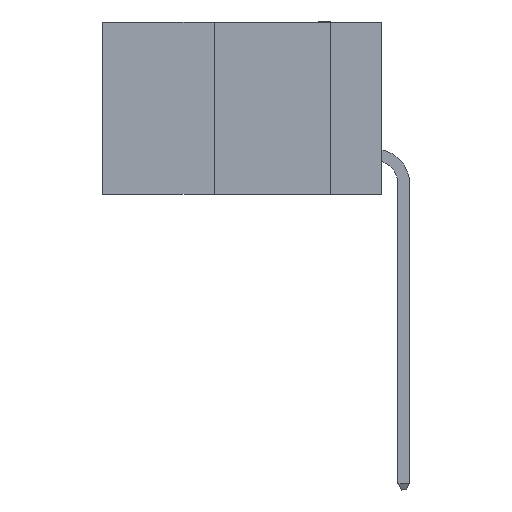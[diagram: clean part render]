
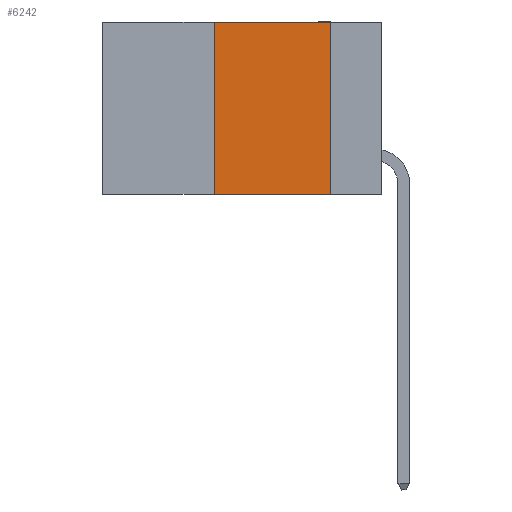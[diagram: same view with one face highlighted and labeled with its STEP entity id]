
A CAD part, left-side view. The second image highlights one B-rep face of the part: STEP entity #6242.
In plain terms, the highlighted planar face has unit normal (-1, 0, 0).
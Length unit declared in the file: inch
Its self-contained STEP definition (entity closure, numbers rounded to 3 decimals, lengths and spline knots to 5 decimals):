
#942 = VECTOR ( 'NONE', #16732, 39.37008 ) ;
#1249 = CARTESIAN_POINT ( 'NONE',  ( 0., 0.11, 0. ) ) ;
#1597 = ORIENTED_EDGE ( 'NONE', *, *, #4186, .T. ) ;
#2632 = PLANE ( 'NONE',  #8872 ) ;
#2743 = VERTEX_POINT ( 'NONE', #24900 ) ;
#3276 = VECTOR ( 'NONE', #30071, 39.37008 ) ;
#3304 = VECTOR ( 'NONE', #22157, 39.37008 ) ;
#4186 = EDGE_CURVE ( 'NONE', #9896, #11917, #15859, .T. ) ;
#4952 = DIRECTION ( 'NONE',  ( 1., 0., 0. ) ) ;
#6058 = VERTEX_POINT ( 'NONE', #1249 ) ;
#6242 = ADVANCED_FACE ( 'NONE', ( #29416 ), #2632, .F. ) ;
#6309 = ORIENTED_EDGE ( 'NONE', *, *, #18442, .F. ) ;
#6749 = CARTESIAN_POINT ( 'NONE',  ( 0., 0.11, -0.37 ) ) ;
#7586 = LINE ( 'NONE', #31676, #942 ) ;
#8872 = AXIS2_PLACEMENT_3D ( 'NONE', #29873, #4952, #22451 ) ;
#9896 = VERTEX_POINT ( 'NONE', #11360 ) ;
#11360 = CARTESIAN_POINT ( 'NONE',  ( 0., 0.36, -0.37 ) ) ;
#11898 = CARTESIAN_POINT ( 'NONE',  ( 0., 0.6, -0.37 ) ) ;
#11917 = VERTEX_POINT ( 'NONE', #6749 ) ;
#15473 = EDGE_CURVE ( 'NONE', #9896, #2743, #7586, .T. ) ;
#15859 = LINE ( 'NONE', #11898, #3304 ) ;
#16732 = DIRECTION ( 'NONE',  ( 0., 0., 1. ) ) ;
#16831 = EDGE_LOOP ( 'NONE', ( #6309, #21452, #23900, #1597 ) ) ;
#18224 = DIRECTION ( 'NONE',  ( 0., 0., -1. ) ) ;
#18442 = EDGE_CURVE ( 'NONE', #6058, #11917, #29910, .T. ) ;
#21452 = ORIENTED_EDGE ( 'NONE', *, *, #31610, .F. ) ;
#22157 = DIRECTION ( 'NONE',  ( 0., -1., 0. ) ) ;
#22451 = DIRECTION ( 'NONE',  ( 0., 0., -1. ) ) ;
#23900 = ORIENTED_EDGE ( 'NONE', *, *, #15473, .F. ) ;
#24900 = CARTESIAN_POINT ( 'NONE',  ( 0., 0.36, 0. ) ) ;
#27537 = CARTESIAN_POINT ( 'NONE',  ( 0., 0.6, 0. ) ) ;
#28454 = CARTESIAN_POINT ( 'NONE',  ( 0., 0.11, 0. ) ) ;
#29416 = FACE_OUTER_BOUND ( 'NONE', #16831, .T. ) ;
#29873 = CARTESIAN_POINT ( 'NONE',  ( 0., 0.6, 0. ) ) ;
#29910 = LINE ( 'NONE', #28454, #30694 ) ;
#30071 = DIRECTION ( 'NONE',  ( 0., -1., 0. ) ) ;
#30694 = VECTOR ( 'NONE', #18224, 39.37008 ) ;
#31610 = EDGE_CURVE ( 'NONE', #2743, #6058, #31836, .T. ) ;
#31676 = CARTESIAN_POINT ( 'NONE',  ( 0., 0.36, 0. ) ) ;
#31836 = LINE ( 'NONE', #27537, #3276 ) ;
